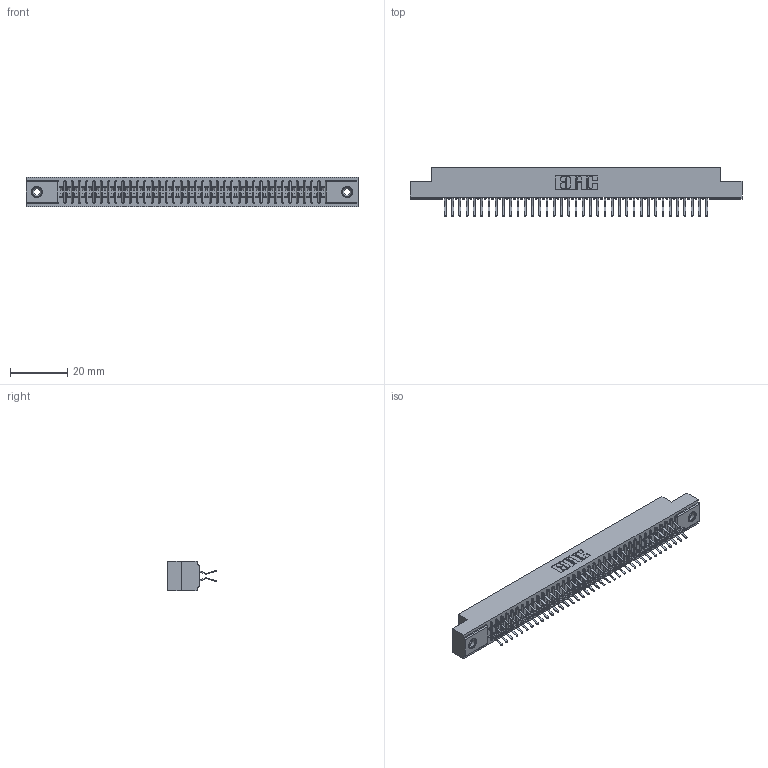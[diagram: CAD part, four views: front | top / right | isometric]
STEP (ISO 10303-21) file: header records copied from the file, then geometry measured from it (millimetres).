
FILE_DESCRIPTION (( 'STEP AP203' ), '1' );
FILE_NAME ('391-074-556-208.STEP', '2018-08-09T14:49:03', ( '' ), ( '' ), 'SwSTEP 2.0', 'SolidWorks 2016', '' );
FILE_SCHEMA (( 'CONFIG_CONTROL_DESIGN' ));
Length unit declared in the file: inch
Products named in the file (4): 341 Part_.156 (3.96) Dia Mounting Holes; 341-292-001_341-292-156; 345-250-001_345-250-003-102; 391-074-556-208
Assembly tree (77 placements, depth 2):
  391-074-556-208
    341 Part_.156 (3.96) Dia Mounting Holes
    341-292-001_341-292-156  x74
    345-250-001_345-250-003-102  x2
Bounding box: 116.2 x 17.07 x 10.16 mm (x, y, z)
Volume: 8593.8 mm3; surface area: 15292.9 mm2
Topology: 77 solids, 77 shells, 5356 faces, 15511 edges, 10058 vertices
Faces by surface type: plane 3060, cylinder 2132, sphere 76, torus 76, cone 12
Entity records: 46769 total; most frequent: CARTESIAN_POINT 7758, ORIENTED_EDGE 7702, DIRECTION 7547, EDGE_CURVE 3851, LINE 3097, VECTOR 3097, VERTEX_POINT 2436, AXIS2_PLACEMENT_3D 2225
